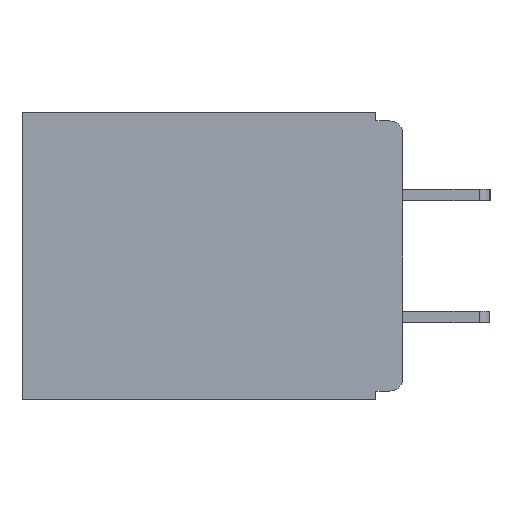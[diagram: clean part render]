
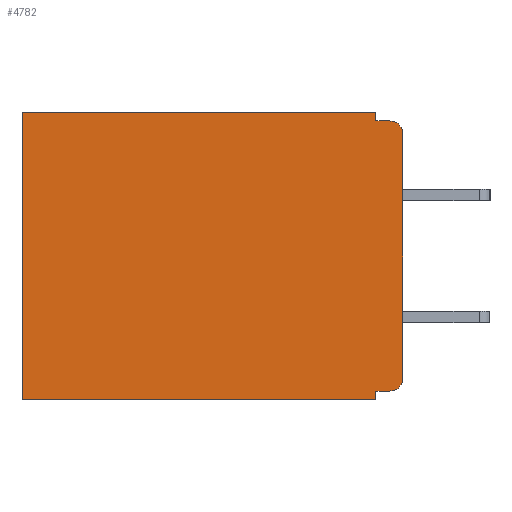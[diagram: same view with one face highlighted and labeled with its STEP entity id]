
A CAD part, left-side view. The second image highlights one B-rep face of the part: STEP entity #4782.
In plain terms, the highlighted planar face has unit normal (-1, 0, 0).
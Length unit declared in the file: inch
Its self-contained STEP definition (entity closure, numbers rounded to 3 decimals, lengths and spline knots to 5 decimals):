
#508 = LINE ( 'NONE', #2973, #23062 ) ;
#585 = ORIENTED_EDGE ( 'NONE', *, *, #6172, .F. ) ;
#752 = DIRECTION ( 'NONE',  ( 1., 0., 0. ) ) ;
#1030 = ORIENTED_EDGE ( 'NONE', *, *, #7635, .T. ) ;
#1100 = DIRECTION ( 'NONE',  ( 0., 1., 0. ) ) ;
#1243 = CIRCLE ( 'NONE', #18501, 0.015 ) ;
#1520 = EDGE_LOOP ( 'NONE', ( #585, #6595, #2619, #3681, #13994, #1030, #1905, #8861, #15655, #13081 ) ) ;
#1905 = ORIENTED_EDGE ( 'NONE', *, *, #19003, .F. ) ;
#2009 = CARTESIAN_POINT ( 'NONE',  ( 0.3, 0.015, -0.025 ) ) ;
#2031 = VERTEX_POINT ( 'NONE', #4382 ) ;
#2137 = LINE ( 'NONE', #17250, #18176 ) ;
#2143 = CARTESIAN_POINT ( 'NONE',  ( 0.3, 0., -0.33 ) ) ;
#2196 = DIRECTION ( 'NONE',  ( 0., 0., -1. ) ) ;
#2543 = DIRECTION ( 'NONE',  ( 0., 0., -1. ) ) ;
#2619 = ORIENTED_EDGE ( 'NONE', *, *, #21247, .F. ) ;
#2636 = VERTEX_POINT ( 'NONE', #6512 ) ;
#2683 = VERTEX_POINT ( 'NONE', #12393 ) ;
#2931 = CARTESIAN_POINT ( 'NONE',  ( 0.3, 0., 0. ) ) ;
#2973 = CARTESIAN_POINT ( 'NONE',  ( 0.3, 0., -0.32 ) ) ;
#3681 = ORIENTED_EDGE ( 'NONE', *, *, #10435, .F. ) ;
#3840 = DIRECTION ( 'NONE',  ( 0., 0., -1. ) ) ;
#4382 = CARTESIAN_POINT ( 'NONE',  ( 0.3, 0.437, 0. ) ) ;
#4782 = ADVANCED_FACE ( 'NONE', ( #17529 ), #6421, .F. ) ;
#5256 = CARTESIAN_POINT ( 'NONE',  ( 0.3, 0., -0.01 ) ) ;
#5495 = VECTOR ( 'NONE', #11282, 39.37008 ) ;
#5857 = VECTOR ( 'NONE', #2543, 39.37008 ) ;
#5922 = AXIS2_PLACEMENT_3D ( 'NONE', #2143, #752, #2196 ) ;
#6075 = CARTESIAN_POINT ( 'NONE',  ( 0.3, 0.031, -0.01 ) ) ;
#6172 = EDGE_CURVE ( 'NONE', #23568, #9847, #18591, .T. ) ;
#6383 = VECTOR ( 'NONE', #19774, 39.37008 ) ;
#6421 = PLANE ( 'NONE',  #5922 ) ;
#6512 = CARTESIAN_POINT ( 'NONE',  ( 0.3, 0.437, -0.33 ) ) ;
#6595 = ORIENTED_EDGE ( 'NONE', *, *, #11496, .T. ) ;
#7635 = EDGE_CURVE ( 'NONE', #2031, #2636, #16707, .T. ) ;
#7880 = EDGE_CURVE ( 'NONE', #21660, #9847, #1243, .T. ) ;
#8135 = VERTEX_POINT ( 'NONE', #6075 ) ;
#8861 = ORIENTED_EDGE ( 'NONE', *, *, #9239, .F. ) ;
#8925 = VECTOR ( 'NONE', #15313, 39.37008 ) ;
#9153 = CARTESIAN_POINT ( 'NONE',  ( 0.3, 0.015, -0.305 ) ) ;
#9239 = EDGE_CURVE ( 'NONE', #15656, #12379, #10363, .T. ) ;
#9543 = EDGE_CURVE ( 'NONE', #14462, #2031, #18060, .T. ) ;
#9847 = VERTEX_POINT ( 'NONE', #21966 ) ;
#10363 = LINE ( 'NONE', #20342, #5495 ) ;
#10435 = EDGE_CURVE ( 'NONE', #14462, #8135, #21690, .T. ) ;
#10960 = DIRECTION ( 'NONE',  ( 0., 0., -1. ) ) ;
#11282 = DIRECTION ( 'NONE',  ( 0., 0., -1. ) ) ;
#11496 = EDGE_CURVE ( 'NONE', #23568, #2683, #12797, .T. ) ;
#11807 = CARTESIAN_POINT ( 'NONE',  ( 0.3, 0.031, 0. ) ) ;
#12379 = VERTEX_POINT ( 'NONE', #19250 ) ;
#12393 = CARTESIAN_POINT ( 'NONE',  ( 0.3, 0.015, -0.01 ) ) ;
#12576 = VECTOR ( 'NONE', #15403, 39.37008 ) ;
#12797 = CIRCLE ( 'NONE', #17834, 0.015 ) ;
#13081 = ORIENTED_EDGE ( 'NONE', *, *, #7880, .T. ) ;
#13820 = CARTESIAN_POINT ( 'NONE',  ( 0.3, 0.031, 0. ) ) ;
#13947 = DIRECTION ( 'NONE',  ( 0., 1., 0. ) ) ;
#13994 = ORIENTED_EDGE ( 'NONE', *, *, #9543, .T. ) ;
#14462 = VERTEX_POINT ( 'NONE', #13820 ) ;
#14790 = DIRECTION ( 'NONE',  ( -1., 0., 0. ) ) ;
#15133 = CARTESIAN_POINT ( 'NONE',  ( 0.3, 0., -0.33 ) ) ;
#15170 = EDGE_CURVE ( 'NONE', #21660, #15656, #508, .T. ) ;
#15313 = DIRECTION ( 'NONE',  ( 0., 0., -1. ) ) ;
#15403 = DIRECTION ( 'NONE',  ( 0., 0., -1. ) ) ;
#15525 = CARTESIAN_POINT ( 'NONE',  ( 0.3, 0.015, -0.32 ) ) ;
#15655 = ORIENTED_EDGE ( 'NONE', *, *, #15170, .F. ) ;
#15656 = VERTEX_POINT ( 'NONE', #22624 ) ;
#16648 = LINE ( 'NONE', #5256, #6383 ) ;
#16707 = LINE ( 'NONE', #20807, #5857 ) ;
#17250 = CARTESIAN_POINT ( 'NONE',  ( 0.3, 0., -0.33 ) ) ;
#17529 = FACE_OUTER_BOUND ( 'NONE', #1520, .T. ) ;
#17834 = AXIS2_PLACEMENT_3D ( 'NONE', #2009, #14790, #3840 ) ;
#18060 = LINE ( 'NONE', #2931, #22251 ) ;
#18176 = VECTOR ( 'NONE', #22605, 39.37008 ) ;
#18501 = AXIS2_PLACEMENT_3D ( 'NONE', #9153, #21829, #10960 ) ;
#18591 = LINE ( 'NONE', #15133, #8925 ) ;
#19003 = EDGE_CURVE ( 'NONE', #12379, #2636, #2137, .T. ) ;
#19250 = CARTESIAN_POINT ( 'NONE',  ( 0.3, 0.031, -0.33 ) ) ;
#19774 = DIRECTION ( 'NONE',  ( 0., -1., 0. ) ) ;
#20342 = CARTESIAN_POINT ( 'NONE',  ( 0.3, 0.031, -0.33 ) ) ;
#20807 = CARTESIAN_POINT ( 'NONE',  ( 0.3, 0.437, -0.33 ) ) ;
#21247 = EDGE_CURVE ( 'NONE', #8135, #2683, #16648, .T. ) ;
#21660 = VERTEX_POINT ( 'NONE', #15525 ) ;
#21690 = LINE ( 'NONE', #11807, #12576 ) ;
#21829 = DIRECTION ( 'NONE',  ( -1., 0., 0. ) ) ;
#21966 = CARTESIAN_POINT ( 'NONE',  ( 0.3, 0., -0.305 ) ) ;
#22251 = VECTOR ( 'NONE', #1100, 39.37008 ) ;
#22605 = DIRECTION ( 'NONE',  ( 0., 1., 0. ) ) ;
#22624 = CARTESIAN_POINT ( 'NONE',  ( 0.3, 0.031, -0.32 ) ) ;
#23062 = VECTOR ( 'NONE', #13947, 39.37008 ) ;
#23568 = VERTEX_POINT ( 'NONE', #23625 ) ;
#23625 = CARTESIAN_POINT ( 'NONE',  ( 0.3, 0., -0.025 ) ) ;
